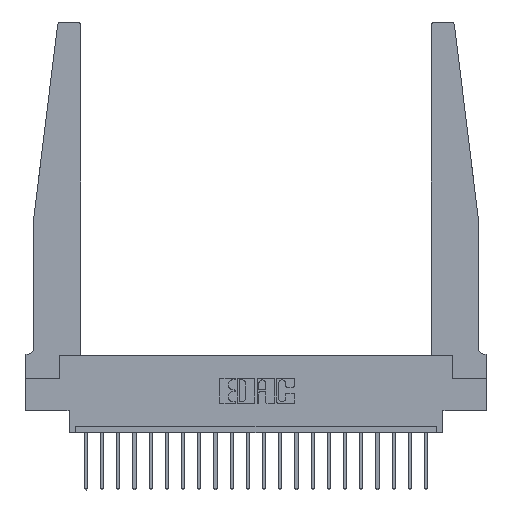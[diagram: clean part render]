
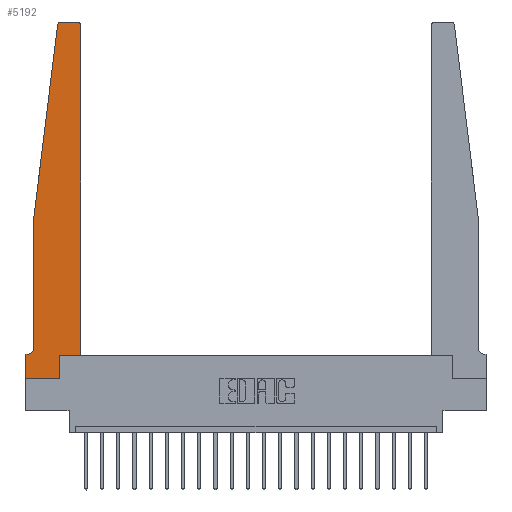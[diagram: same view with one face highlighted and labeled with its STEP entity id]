
A CAD part, top view. The second image highlights one B-rep face of the part: STEP entity #5192.
In plain terms, the highlighted planar face has unit normal (0, 0, 1).
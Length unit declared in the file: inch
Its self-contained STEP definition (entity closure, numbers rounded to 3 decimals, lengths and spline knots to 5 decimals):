
#520 = CARTESIAN_POINT ( 'NONE',  ( 0.065, 1.25, 0.37 ) ) ;
#629 = EDGE_CURVE ( 'NONE', #13708, #740, #8111, .T. ) ;
#661 = LINE ( 'NONE', #15397, #4019 ) ;
#740 = VERTEX_POINT ( 'NONE', #11173 ) ;
#894 = DIRECTION ( 'NONE',  ( 1., 0., 0. ) ) ;
#951 = CARTESIAN_POINT ( 'NONE',  ( 0.25, 2.75, 0.37 ) ) ;
#1346 = VECTOR ( 'NONE', #6765, 39.37008 ) ;
#1395 = CARTESIAN_POINT ( 'NONE',  ( 0.065, 0.1875, 0.37 ) ) ;
#1799 = DIRECTION ( 'NONE',  ( 1., 0., 0. ) ) ;
#1911 = CARTESIAN_POINT ( 'NONE',  ( 0., 0., 0.37 ) ) ;
#2057 = DIRECTION ( 'NONE',  ( 0., -1., 0. ) ) ;
#2385 = VECTOR ( 'NONE', #5404, 39.37008 ) ;
#2654 = AXIS2_PLACEMENT_3D ( 'NONE', #17632, #6050, #14195 ) ;
#2702 = CARTESIAN_POINT ( 'NONE',  ( 0.2605, 0.18, 0.37 ) ) ;
#2992 = ORIENTED_EDGE ( 'NONE', *, *, #629, .T. ) ;
#3277 = ORIENTED_EDGE ( 'NONE', *, *, #18271, .T. ) ;
#3456 = VERTEX_POINT ( 'NONE', #2702 ) ;
#3593 = ORIENTED_EDGE ( 'NONE', *, *, #12913, .T. ) ;
#3926 = VECTOR ( 'NONE', #6155, 39.37008 ) ;
#4019 = VECTOR ( 'NONE', #12138, 39.37008 ) ;
#4600 = DIRECTION ( 'NONE',  ( 0., 1., 0. ) ) ;
#4932 = ORIENTED_EDGE ( 'NONE', *, *, #12522, .T. ) ;
#4936 = CARTESIAN_POINT ( 'NONE',  ( 0., 0.1875, 0.37 ) ) ;
#5084 = VERTEX_POINT ( 'NONE', #6220 ) ;
#5121 = LINE ( 'NONE', #1911, #19250 ) ;
#5171 = VERTEX_POINT ( 'NONE', #21071 ) ;
#5192 = ADVANCED_FACE ( 'NONE', ( #9608 ), #9768, .T. ) ;
#5404 = DIRECTION ( 'NONE',  ( 1., 0., 0. ) ) ;
#5480 = ORIENTED_EDGE ( 'NONE', *, *, #10522, .T. ) ;
#5581 = CIRCLE ( 'NONE', #7003, 0.03 ) ;
#5690 = CARTESIAN_POINT ( 'NONE',  ( 0.425, 2.72, 0.37 ) ) ;
#5692 = LINE ( 'NONE', #15991, #3926 ) ;
#6050 = DIRECTION ( 'NONE',  ( 0., 0., 1. ) ) ;
#6093 = ORIENTED_EDGE ( 'NONE', *, *, #19282, .T. ) ;
#6155 = DIRECTION ( 'NONE',  ( 0., 1., 0. ) ) ;
#6220 = CARTESIAN_POINT ( 'NONE',  ( 0.395, 2.75, 0.37 ) ) ;
#6556 = ORIENTED_EDGE ( 'NONE', *, *, #10733, .T. ) ;
#6701 = EDGE_LOOP ( 'NONE', ( #6556, #6093, #5480, #10704, #2992, #3593, #12910, #16094, #3277, #4932, #11851, #12478 ) ) ;
#6765 = DIRECTION ( 'NONE',  ( -1., 0., 0. ) ) ;
#6796 = DIRECTION ( 'NONE',  ( -0.122, -0.992, 0. ) ) ;
#7003 = AXIS2_PLACEMENT_3D ( 'NONE', #9115, #14207, #894 ) ;
#8111 = CIRCLE ( 'NONE', #17325, 0.05 ) ;
#8198 = CARTESIAN_POINT ( 'NONE',  ( 0.425, 0.18, 0.37 ) ) ;
#8374 = DIRECTION ( 'NONE',  ( 1., 0., 0. ) ) ;
#8480 = CARTESIAN_POINT ( 'NONE',  ( 0.27653, 2.75, 0.37 ) ) ;
#8643 = EDGE_CURVE ( 'NONE', #19202, #5084, #5581, .T. ) ;
#8693 = EDGE_CURVE ( 'NONE', #18884, #19202, #16689, .T. ) ;
#8763 = CIRCLE ( 'NONE', #2654, 0.03 ) ;
#8930 = CARTESIAN_POINT ( 'NONE',  ( 0.065, 0.2375, 0.37 ) ) ;
#9115 = CARTESIAN_POINT ( 'NONE',  ( 0.395, 2.72, 0.37 ) ) ;
#9279 = VERTEX_POINT ( 'NONE', #17655 ) ;
#9608 = FACE_OUTER_BOUND ( 'NONE', #6701, .T. ) ;
#9757 = EDGE_CURVE ( 'NONE', #9279, #14949, #661, .T. ) ;
#9768 = PLANE ( 'NONE',  #11679 ) ;
#9924 = DIRECTION ( 'NONE',  ( 0., 0., 1. ) ) ;
#9925 = LINE ( 'NONE', #11782, #10435 ) ;
#10140 = CARTESIAN_POINT ( 'NONE',  ( 0., 0., 0.37 ) ) ;
#10435 = VECTOR ( 'NONE', #6796, 39.37008 ) ;
#10522 = EDGE_CURVE ( 'NONE', #5171, #20119, #9925, .T. ) ;
#10704 = ORIENTED_EDGE ( 'NONE', *, *, #14197, .T. ) ;
#10733 = EDGE_CURVE ( 'NONE', #5084, #14375, #15824, .T. ) ;
#11170 = CARTESIAN_POINT ( 'NONE',  ( 0.065, 1.25, 0.37 ) ) ;
#11173 = CARTESIAN_POINT ( 'NONE',  ( 0.015, 0.1875, 0.37 ) ) ;
#11423 = CARTESIAN_POINT ( 'NONE',  ( 0.425, 0.18, 0.37 ) ) ;
#11679 = AXIS2_PLACEMENT_3D ( 'NONE', #4936, #9924, #1799 ) ;
#11782 = CARTESIAN_POINT ( 'NONE',  ( 0.065, 1.25, 0.37 ) ) ;
#11844 = LINE ( 'NONE', #520, #19507 ) ;
#11851 = ORIENTED_EDGE ( 'NONE', *, *, #8693, .T. ) ;
#12130 = VERTEX_POINT ( 'NONE', #16005 ) ;
#12138 = DIRECTION ( 'NONE',  ( 0., -1., 0. ) ) ;
#12478 = ORIENTED_EDGE ( 'NONE', *, *, #8643, .T. ) ;
#12522 = EDGE_CURVE ( 'NONE', #3456, #18884, #20616, .T. ) ;
#12528 = DIRECTION ( 'NONE',  ( 0., 0., -1. ) ) ;
#12910 = ORIENTED_EDGE ( 'NONE', *, *, #9757, .T. ) ;
#12913 = EDGE_CURVE ( 'NONE', #740, #9279, #14480, .T. ) ;
#13708 = VERTEX_POINT ( 'NONE', #8930 ) ;
#14195 = DIRECTION ( 'NONE',  ( 1., 0., 0. ) ) ;
#14197 = EDGE_CURVE ( 'NONE', #20119, #13708, #11844, .T. ) ;
#14207 = DIRECTION ( 'NONE',  ( 0., 0., 1. ) ) ;
#14375 = VERTEX_POINT ( 'NONE', #8480 ) ;
#14480 = LINE ( 'NONE', #1395, #1346 ) ;
#14949 = VERTEX_POINT ( 'NONE', #10140 ) ;
#15307 = VECTOR ( 'NONE', #15790, 39.37008 ) ;
#15397 = CARTESIAN_POINT ( 'NONE',  ( 0., 0., 0.37 ) ) ;
#15790 = DIRECTION ( 'NONE',  ( -1., 0., 0. ) ) ;
#15824 = LINE ( 'NONE', #951, #15307 ) ;
#15991 = CARTESIAN_POINT ( 'NONE',  ( 0.2605, 0.18, 0.37 ) ) ;
#16005 = CARTESIAN_POINT ( 'NONE',  ( 0.2605, 0., 0.37 ) ) ;
#16094 = ORIENTED_EDGE ( 'NONE', *, *, #19551, .T. ) ;
#16689 = LINE ( 'NONE', #8198, #18197 ) ;
#17325 = AXIS2_PLACEMENT_3D ( 'NONE', #20471, #12528, #17466 ) ;
#17466 = DIRECTION ( 'NONE',  ( -1., 0., 0. ) ) ;
#17632 = CARTESIAN_POINT ( 'NONE',  ( 0.27653, 2.72, 0.37 ) ) ;
#17655 = CARTESIAN_POINT ( 'NONE',  ( 0., 0.1875, 0.37 ) ) ;
#18197 = VECTOR ( 'NONE', #4600, 39.37008 ) ;
#18271 = EDGE_CURVE ( 'NONE', #12130, #3456, #5692, .T. ) ;
#18495 = CARTESIAN_POINT ( 'NONE',  ( 0.425, 0.18, 0.37 ) ) ;
#18884 = VERTEX_POINT ( 'NONE', #11423 ) ;
#19202 = VERTEX_POINT ( 'NONE', #5690 ) ;
#19250 = VECTOR ( 'NONE', #8374, 39.37008 ) ;
#19282 = EDGE_CURVE ( 'NONE', #14375, #5171, #8763, .T. ) ;
#19507 = VECTOR ( 'NONE', #2057, 39.37008 ) ;
#19551 = EDGE_CURVE ( 'NONE', #14949, #12130, #5121, .T. ) ;
#20119 = VERTEX_POINT ( 'NONE', #11170 ) ;
#20471 = CARTESIAN_POINT ( 'NONE',  ( 0.015, 0.2375, 0.37 ) ) ;
#20616 = LINE ( 'NONE', #18495, #2385 ) ;
#21071 = CARTESIAN_POINT ( 'NONE',  ( 0.24675, 2.72367, 0.37 ) ) ;
